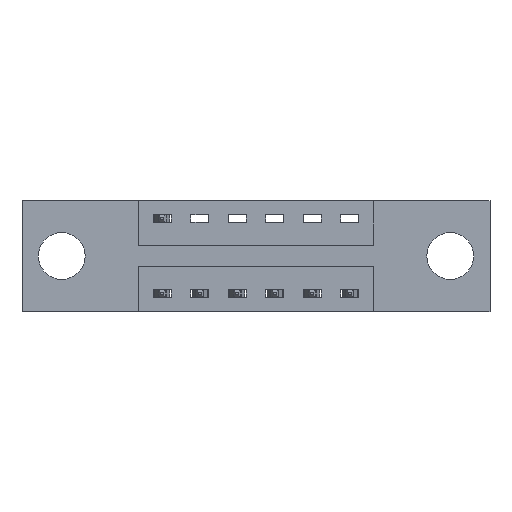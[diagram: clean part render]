
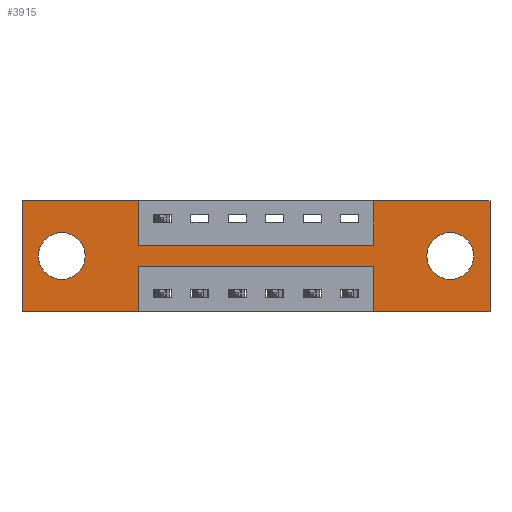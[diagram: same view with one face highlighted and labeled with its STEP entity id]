
A CAD part, front view. The second image highlights one B-rep face of the part: STEP entity #3915.
In plain terms, the highlighted planar face has unit normal (0, -1, 0).
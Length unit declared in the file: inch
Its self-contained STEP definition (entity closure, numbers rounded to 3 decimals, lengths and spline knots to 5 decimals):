
#21 = DIRECTION ( 'NONE',  ( 0., 0., -1. ) ) ;
#28 = CARTESIAN_POINT ( 'NONE',  ( 1.1725, 0., -0.15 ) ) ;
#39 = AXIS2_PLACEMENT_3D ( 'NONE', #3061, #3697, #7246 ) ;
#43 = VECTOR ( 'NONE', #885, 39.37008 ) ;
#85 = ORIENTED_EDGE ( 'NONE', *, *, #5772, .F. ) ;
#94 = ORIENTED_EDGE ( 'NONE', *, *, #1729, .F. ) ;
#164 = CARTESIAN_POINT ( 'NONE',  ( 0.1325, 0., -0.185 ) ) ;
#236 = VERTEX_POINT ( 'NONE', #3118 ) ;
#243 = ORIENTED_EDGE ( 'NONE', *, *, #830, .T. ) ;
#246 = VERTEX_POINT ( 'NONE', #3570 ) ;
#254 = EDGE_CURVE ( 'NONE', #921, #956, #4069, .T. ) ;
#260 = AXIS2_PLACEMENT_3D ( 'NONE', #2347, #6867, #3004 ) ;
#287 = EDGE_CURVE ( 'NONE', #3526, #236, #3668, .T. ) ;
#311 = ORIENTED_EDGE ( 'NONE', *, *, #4764, .F. ) ;
#536 = ORIENTED_EDGE ( 'NONE', *, *, #1545, .F. ) ;
#575 = ORIENTED_EDGE ( 'NONE', *, *, #5593, .F. ) ;
#617 = VERTEX_POINT ( 'NONE', #6984 ) ;
#662 = ORIENTED_EDGE ( 'NONE', *, *, #2097, .F. ) ;
#805 = AXIS2_PLACEMENT_3D ( 'NONE', #6421, #3233, #7770 ) ;
#830 = EDGE_CURVE ( 'NONE', #236, #3526, #8310, .T. ) ;
#872 = LINE ( 'NONE', #2742, #4255 ) ;
#879 = EDGE_CURVE ( 'NONE', #3640, #3389, #872, .T. ) ;
#885 = DIRECTION ( 'NONE',  ( 1., 0., 0. ) ) ;
#921 = VERTEX_POINT ( 'NONE', #5183 ) ;
#952 = FACE_BOUND ( 'NONE', #1639, .T. ) ;
#956 = VERTEX_POINT ( 'NONE', #4365 ) ;
#974 = CARTESIAN_POINT ( 'NONE',  ( 0., 0., 0. ) ) ;
#1188 = EDGE_CURVE ( 'NONE', #956, #4898, #5048, .T. ) ;
#1189 = PLANE ( 'NONE',  #805 ) ;
#1192 = VECTOR ( 'NONE', #7935, 39.37008 ) ;
#1195 = ORIENTED_EDGE ( 'NONE', *, *, #1188, .F. ) ;
#1258 = ORIENTED_EDGE ( 'NONE', *, *, #254, .F. ) ;
#1268 = VERTEX_POINT ( 'NONE', #5476 ) ;
#1545 = EDGE_CURVE ( 'NONE', #8638, #5254, #6947, .T. ) ;
#1622 = VECTOR ( 'NONE', #2730, 39.37008 ) ;
#1639 = EDGE_LOOP ( 'NONE', ( #1698, #8642 ) ) ;
#1641 = CARTESIAN_POINT ( 'NONE',  ( 1.56, 0., 0. ) ) ;
#1698 = ORIENTED_EDGE ( 'NONE', *, *, #4741, .T. ) ;
#1729 = EDGE_CURVE ( 'NONE', #7225, #1777, #8579, .T. ) ;
#1777 = VERTEX_POINT ( 'NONE', #6230 ) ;
#1780 = CARTESIAN_POINT ( 'NONE',  ( 0.3875, 0., 0. ) ) ;
#1837 = DIRECTION ( 'NONE',  ( -1., 0., 0. ) ) ;
#1870 = DIRECTION ( 'NONE',  ( 0., 0., -1. ) ) ;
#1927 = LINE ( 'NONE', #1641, #5222 ) ;
#2041 = ORIENTED_EDGE ( 'NONE', *, *, #2822, .F. ) ;
#2068 = VERTEX_POINT ( 'NONE', #7909 ) ;
#2097 = EDGE_CURVE ( 'NONE', #4898, #6489, #8572, .T. ) ;
#2162 = CARTESIAN_POINT ( 'NONE',  ( 0.1325, 0., -0.263 ) ) ;
#2329 = VECTOR ( 'NONE', #2600, 39.37008 ) ;
#2347 = CARTESIAN_POINT ( 'NONE',  ( 1.4275, 0., -0.185 ) ) ;
#2378 = FACE_BOUND ( 'NONE', #3285, .T. ) ;
#2508 = DIRECTION ( 'NONE',  ( 0., 0., 1. ) ) ;
#2559 = ORIENTED_EDGE ( 'NONE', *, *, #879, .F. ) ;
#2600 = DIRECTION ( 'NONE',  ( 1., 0., 0. ) ) ;
#2671 = DIRECTION ( 'NONE',  ( 0., 0., 1. ) ) ;
#2715 = CARTESIAN_POINT ( 'NONE',  ( 0., 0., 0. ) ) ;
#2730 = DIRECTION ( 'NONE',  ( 0., 0., 1. ) ) ;
#2742 = CARTESIAN_POINT ( 'NONE',  ( 0., 0., -0.37 ) ) ;
#2822 = EDGE_CURVE ( 'NONE', #3389, #921, #5137, .T. ) ;
#2924 = AXIS2_PLACEMENT_3D ( 'NONE', #8026, #4149, #21 ) ;
#3004 = DIRECTION ( 'NONE',  ( 0., 0., -1. ) ) ;
#3025 = CARTESIAN_POINT ( 'NONE',  ( 0.3875, 0., -0.37 ) ) ;
#3061 = CARTESIAN_POINT ( 'NONE',  ( 0.1325, 0., -0.185 ) ) ;
#3062 = EDGE_LOOP ( 'NONE', ( #7328, #4187, #85, #94, #311, #536, #575, #662, #1195, #1258, #2041, #2559 ) ) ;
#3118 = CARTESIAN_POINT ( 'NONE',  ( 0.1325, 0., -0.107 ) ) ;
#3233 = DIRECTION ( 'NONE',  ( 0., -1., 0. ) ) ;
#3285 = EDGE_LOOP ( 'NONE', ( #243, #5601 ) ) ;
#3389 = VERTEX_POINT ( 'NONE', #5309 ) ;
#3403 = CARTESIAN_POINT ( 'NONE',  ( 0.3875, 0., -0.15 ) ) ;
#3476 = VECTOR ( 'NONE', #6959, 39.37008 ) ;
#3485 = CARTESIAN_POINT ( 'NONE',  ( 1.56, 0., 0. ) ) ;
#3515 = CARTESIAN_POINT ( 'NONE',  ( 1.56, 0., -0.37 ) ) ;
#3526 = VERTEX_POINT ( 'NONE', #2162 ) ;
#3541 = VECTOR ( 'NONE', #1870, 39.37008 ) ;
#3545 = CIRCLE ( 'NONE', #2924, 0.078 ) ;
#3564 = VECTOR ( 'NONE', #3694, 39.37008 ) ;
#3570 = CARTESIAN_POINT ( 'NONE',  ( 1.1725, 0., -0.22 ) ) ;
#3612 = CARTESIAN_POINT ( 'NONE',  ( 0., 0., -0.37 ) ) ;
#3640 = VERTEX_POINT ( 'NONE', #5544 ) ;
#3668 = CIRCLE ( 'NONE', #39, 0.078 ) ;
#3671 = DIRECTION ( 'NONE',  ( 0., 0., -1. ) ) ;
#3694 = DIRECTION ( 'NONE',  ( 0., 0., -1. ) ) ;
#3697 = DIRECTION ( 'NONE',  ( 0., 1., 0. ) ) ;
#3714 = CIRCLE ( 'NONE', #260, 0.078 ) ;
#3915 = ADVANCED_FACE ( 'NONE', ( #952, #2378, #5800 ), #1189, .T. ) ;
#4069 = LINE ( 'NONE', #2715, #2329 ) ;
#4149 = DIRECTION ( 'NONE',  ( 0., 1., 0. ) ) ;
#4187 = ORIENTED_EDGE ( 'NONE', *, *, #6192, .F. ) ;
#4255 = VECTOR ( 'NONE', #1837, 39.37008 ) ;
#4365 = CARTESIAN_POINT ( 'NONE',  ( 0.3875, 0., 0. ) ) ;
#4741 = EDGE_CURVE ( 'NONE', #617, #2068, #3714, .T. ) ;
#4764 = EDGE_CURVE ( 'NONE', #5254, #7225, #1927, .T. ) ;
#4797 = LINE ( 'NONE', #6519, #8250 ) ;
#4898 = VERTEX_POINT ( 'NONE', #5702 ) ;
#4903 = LINE ( 'NONE', #5714, #6185 ) ;
#4940 = VECTOR ( 'NONE', #6802, 39.37008 ) ;
#5048 = LINE ( 'NONE', #1780, #3541 ) ;
#5137 = LINE ( 'NONE', #8565, #1622 ) ;
#5183 = CARTESIAN_POINT ( 'NONE',  ( 0., 0., 0. ) ) ;
#5222 = VECTOR ( 'NONE', #3671, 39.37008 ) ;
#5254 = VERTEX_POINT ( 'NONE', #3485 ) ;
#5278 = LINE ( 'NONE', #3025, #3564 ) ;
#5309 = CARTESIAN_POINT ( 'NONE',  ( 0., 0., -0.37 ) ) ;
#5476 = CARTESIAN_POINT ( 'NONE',  ( 0.3875, 0., -0.22 ) ) ;
#5544 = CARTESIAN_POINT ( 'NONE',  ( 0.3875, 0., -0.37 ) ) ;
#5593 = EDGE_CURVE ( 'NONE', #6489, #8638, #4903, .T. ) ;
#5595 = CARTESIAN_POINT ( 'NONE',  ( 1.1725, 0., 0. ) ) ;
#5601 = ORIENTED_EDGE ( 'NONE', *, *, #287, .T. ) ;
#5702 = CARTESIAN_POINT ( 'NONE',  ( 0.3875, 0., -0.15 ) ) ;
#5714 = CARTESIAN_POINT ( 'NONE',  ( 1.1725, 0., 0. ) ) ;
#5735 = AXIS2_PLACEMENT_3D ( 'NONE', #164, #7841, #6406 ) ;
#5772 = EDGE_CURVE ( 'NONE', #1777, #246, #4797, .T. ) ;
#5800 = FACE_OUTER_BOUND ( 'NONE', #3062, .T. ) ;
#6185 = VECTOR ( 'NONE', #2508, 39.37008 ) ;
#6192 = EDGE_CURVE ( 'NONE', #246, #1268, #6895, .T. ) ;
#6230 = CARTESIAN_POINT ( 'NONE',  ( 1.1725, 0., -0.37 ) ) ;
#6296 = CARTESIAN_POINT ( 'NONE',  ( 0.3875, 0., -0.22 ) ) ;
#6406 = DIRECTION ( 'NONE',  ( 0., 0., 1. ) ) ;
#6421 = CARTESIAN_POINT ( 'NONE',  ( 0., 0., -0.37 ) ) ;
#6489 = VERTEX_POINT ( 'NONE', #28 ) ;
#6519 = CARTESIAN_POINT ( 'NONE',  ( 1.1725, 0., -0.37 ) ) ;
#6802 = DIRECTION ( 'NONE',  ( -1., 0., 0. ) ) ;
#6867 = DIRECTION ( 'NONE',  ( 0., 1., 0. ) ) ;
#6895 = LINE ( 'NONE', #6296, #3476 ) ;
#6947 = LINE ( 'NONE', #974, #43 ) ;
#6959 = DIRECTION ( 'NONE',  ( -1., 0., 0. ) ) ;
#6984 = CARTESIAN_POINT ( 'NONE',  ( 1.4275, 0., -0.107 ) ) ;
#7225 = VERTEX_POINT ( 'NONE', #3515 ) ;
#7246 = DIRECTION ( 'NONE',  ( 0., 0., 1. ) ) ;
#7328 = ORIENTED_EDGE ( 'NONE', *, *, #7378, .F. ) ;
#7378 = EDGE_CURVE ( 'NONE', #1268, #3640, #5278, .T. ) ;
#7770 = DIRECTION ( 'NONE',  ( 0., 0., -1. ) ) ;
#7841 = DIRECTION ( 'NONE',  ( 0., 1., 0. ) ) ;
#7909 = CARTESIAN_POINT ( 'NONE',  ( 1.4275, 0., -0.263 ) ) ;
#7935 = DIRECTION ( 'NONE',  ( 1., 0., 0. ) ) ;
#8026 = CARTESIAN_POINT ( 'NONE',  ( 1.4275, 0., -0.185 ) ) ;
#8250 = VECTOR ( 'NONE', #2671, 39.37008 ) ;
#8310 = CIRCLE ( 'NONE', #5735, 0.078 ) ;
#8459 = EDGE_CURVE ( 'NONE', #2068, #617, #3545, .T. ) ;
#8565 = CARTESIAN_POINT ( 'NONE',  ( 0., 0., 0. ) ) ;
#8572 = LINE ( 'NONE', #3403, #1192 ) ;
#8579 = LINE ( 'NONE', #3612, #4940 ) ;
#8638 = VERTEX_POINT ( 'NONE', #5595 ) ;
#8642 = ORIENTED_EDGE ( 'NONE', *, *, #8459, .T. ) ;
